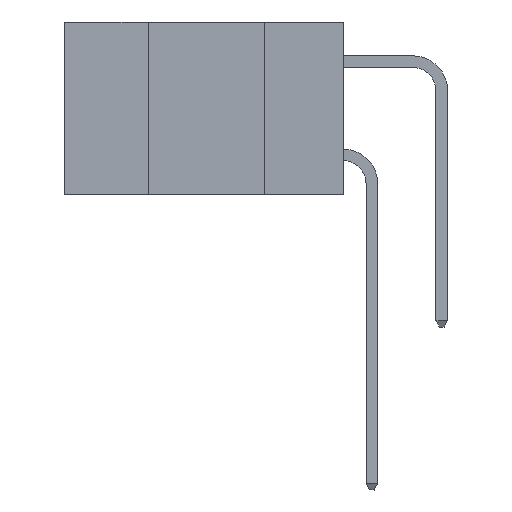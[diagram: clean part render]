
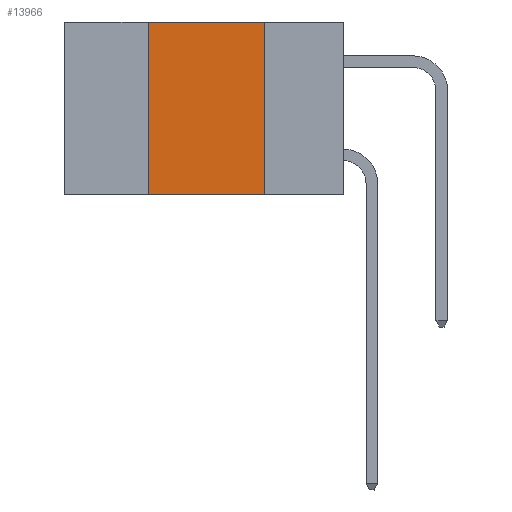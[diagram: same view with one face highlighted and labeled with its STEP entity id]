
A CAD part, left-side view. The second image highlights one B-rep face of the part: STEP entity #13966.
In plain terms, the highlighted planar face has unit normal (-1, 0, 0).
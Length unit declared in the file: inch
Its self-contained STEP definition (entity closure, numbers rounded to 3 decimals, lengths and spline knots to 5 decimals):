
#316 = EDGE_LOOP ( 'NONE', ( #8671, #1225, #13715, #13576 ) ) ;
#717 = EDGE_CURVE ( 'NONE', #4744, #12030, #13974, .T. ) ;
#1225 = ORIENTED_EDGE ( 'NONE', *, *, #717, .F. ) ;
#1709 = VERTEX_POINT ( 'NONE', #6288 ) ;
#1894 = DIRECTION ( 'NONE',  ( 0., -1., 0. ) ) ;
#2119 = CARTESIAN_POINT ( 'NONE',  ( 0., 0.6, -0.37 ) ) ;
#3263 = CARTESIAN_POINT ( 'NONE',  ( 0., 0.17, -0.37 ) ) ;
#3736 = VECTOR ( 'NONE', #4328, 39.37008 ) ;
#4328 = DIRECTION ( 'NONE',  ( 0., 0., 1. ) ) ;
#4475 = CARTESIAN_POINT ( 'NONE',  ( 0., 0.6, 0. ) ) ;
#4744 = VERTEX_POINT ( 'NONE', #14368 ) ;
#5362 = DIRECTION ( 'NONE',  ( 0., -1., 0. ) ) ;
#5695 = CARTESIAN_POINT ( 'NONE',  ( 0., 0.17, 0. ) ) ;
#5721 = PLANE ( 'NONE',  #7029 ) ;
#5796 = DIRECTION ( 'NONE',  ( 1., 0., 0. ) ) ;
#6288 = CARTESIAN_POINT ( 'NONE',  ( 0., 0.42, -0.37 ) ) ;
#6549 = CARTESIAN_POINT ( 'NONE',  ( 0., 0.17, -0.37 ) ) ;
#6792 = EDGE_CURVE ( 'NONE', #12030, #8519, #11198, .T. ) ;
#6848 = DIRECTION ( 'NONE',  ( 0., 0., -1. ) ) ;
#7029 = AXIS2_PLACEMENT_3D ( 'NONE', #4475, #5796, #6848 ) ;
#7066 = VECTOR ( 'NONE', #11055, 39.37008 ) ;
#8519 = VERTEX_POINT ( 'NONE', #3263 ) ;
#8671 = ORIENTED_EDGE ( 'NONE', *, *, #6792, .F. ) ;
#8918 = VECTOR ( 'NONE', #5362, 39.37008 ) ;
#10095 = CARTESIAN_POINT ( 'NONE',  ( 0., 0.42, -0.37 ) ) ;
#10191 = FACE_OUTER_BOUND ( 'NONE', #316, .T. ) ;
#10937 = VECTOR ( 'NONE', #1894, 39.37008 ) ;
#11055 = DIRECTION ( 'NONE',  ( 0., 0., -1. ) ) ;
#11198 = LINE ( 'NONE', #6549, #7066 ) ;
#12030 = VERTEX_POINT ( 'NONE', #5695 ) ;
#12941 = CARTESIAN_POINT ( 'NONE',  ( 0., 0.6, 0. ) ) ;
#13233 = EDGE_CURVE ( 'NONE', #1709, #4744, #14409, .T. ) ;
#13576 = ORIENTED_EDGE ( 'NONE', *, *, #14504, .T. ) ;
#13715 = ORIENTED_EDGE ( 'NONE', *, *, #13233, .F. ) ;
#13966 = ADVANCED_FACE ( 'NONE', ( #10191 ), #5721, .F. ) ;
#13974 = LINE ( 'NONE', #12941, #10937 ) ;
#14333 = LINE ( 'NONE', #2119, #8918 ) ;
#14368 = CARTESIAN_POINT ( 'NONE',  ( 0., 0.42, 0. ) ) ;
#14409 = LINE ( 'NONE', #10095, #3736 ) ;
#14504 = EDGE_CURVE ( 'NONE', #1709, #8519, #14333, .T. ) ;
